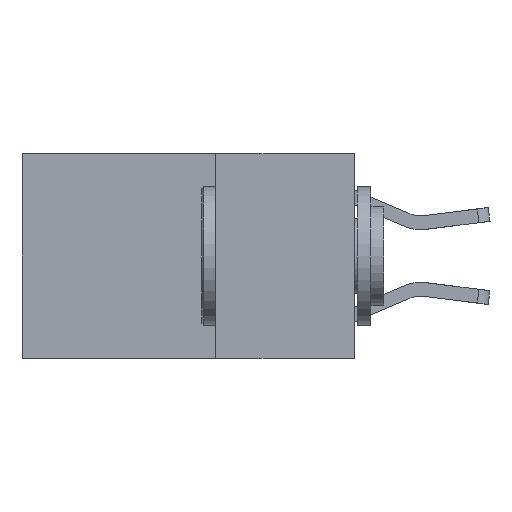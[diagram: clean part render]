
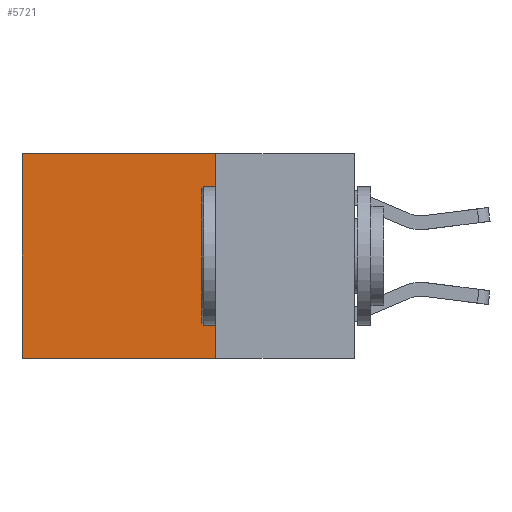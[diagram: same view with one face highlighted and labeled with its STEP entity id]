
A CAD part, left-side view. The second image highlights one B-rep face of the part: STEP entity #5721.
In plain terms, the highlighted planar face has unit normal (-1, 0, 0).
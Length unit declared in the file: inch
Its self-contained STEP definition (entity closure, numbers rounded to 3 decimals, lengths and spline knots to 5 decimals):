
#12 = CARTESIAN_POINT ( 'NONE',  ( 0.2625, 0.25, 0. ) ) ;
#172 = ORIENTED_EDGE ( 'NONE', *, *, #3624, .T. ) ;
#254 = DIRECTION ( 'NONE',  ( 0., 1., 0. ) ) ;
#304 = ORIENTED_EDGE ( 'NONE', *, *, #11031, .T. ) ;
#807 = VECTOR ( 'NONE', #2389, 39.37008 ) ;
#972 = PLANE ( 'NONE',  #9496 ) ;
#1049 = ORIENTED_EDGE ( 'NONE', *, *, #3937, .F. ) ;
#1242 = VERTEX_POINT ( 'NONE', #10713 ) ;
#1566 = CARTESIAN_POINT ( 'NONE',  ( 0.2625, 0.25, 0. ) ) ;
#1579 = VECTOR ( 'NONE', #7042, 39.37008 ) ;
#2389 = DIRECTION ( 'NONE',  ( 0., 0., -1. ) ) ;
#2767 = CARTESIAN_POINT ( 'NONE',  ( 0.2625, 0.25, 0. ) ) ;
#2915 = LINE ( 'NONE', #10815, #7532 ) ;
#3543 = CARTESIAN_POINT ( 'NONE',  ( 0.2625, 0.6, -0.37 ) ) ;
#3624 = EDGE_CURVE ( 'NONE', #3730, #3781, #2915, .T. ) ;
#3730 = VERTEX_POINT ( 'NONE', #1566 ) ;
#3781 = VERTEX_POINT ( 'NONE', #8099 ) ;
#3887 = LINE ( 'NONE', #2767, #1579 ) ;
#3937 = EDGE_CURVE ( 'NONE', #3730, #1242, #3887, .T. ) ;
#4603 = EDGE_LOOP ( 'NONE', ( #304, #9265, #1049, #172 ) ) ;
#4653 = VERTEX_POINT ( 'NONE', #3543 ) ;
#5116 = CARTESIAN_POINT ( 'NONE',  ( 0.2625, 0.25, -0.37 ) ) ;
#5721 = ADVANCED_FACE ( 'NONE', ( #7781 ), #972, .F. ) ;
#5920 = CARTESIAN_POINT ( 'NONE',  ( 0.2625, 0.6, 0. ) ) ;
#6079 = DIRECTION ( 'NONE',  ( 1., 0., 0. ) ) ;
#6345 = EDGE_CURVE ( 'NONE', #1242, #4653, #10990, .T. ) ;
#6658 = LINE ( 'NONE', #5920, #807 ) ;
#7042 = DIRECTION ( 'NONE',  ( 0., 0., -1. ) ) ;
#7532 = VECTOR ( 'NONE', #254, 39.37008 ) ;
#7781 = FACE_OUTER_BOUND ( 'NONE', #4603, .T. ) ;
#8099 = CARTESIAN_POINT ( 'NONE',  ( 0.2625, 0.6, 0. ) ) ;
#8735 = DIRECTION ( 'NONE',  ( 0., 0., -1. ) ) ;
#9265 = ORIENTED_EDGE ( 'NONE', *, *, #6345, .F. ) ;
#9496 = AXIS2_PLACEMENT_3D ( 'NONE', #12, #6079, #8735 ) ;
#10277 = VECTOR ( 'NONE', #10929, 39.37008 ) ;
#10713 = CARTESIAN_POINT ( 'NONE',  ( 0.2625, 0.25, -0.37 ) ) ;
#10815 = CARTESIAN_POINT ( 'NONE',  ( 0.2625, 0.25, 0. ) ) ;
#10929 = DIRECTION ( 'NONE',  ( 0., 1., 0. ) ) ;
#10990 = LINE ( 'NONE', #5116, #10277 ) ;
#11031 = EDGE_CURVE ( 'NONE', #3781, #4653, #6658, .T. ) ;
